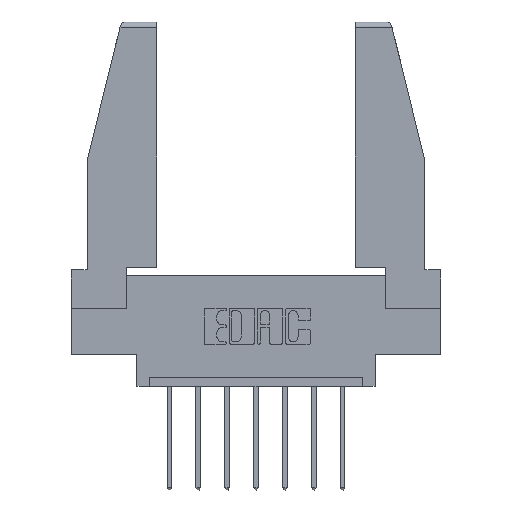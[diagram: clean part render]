
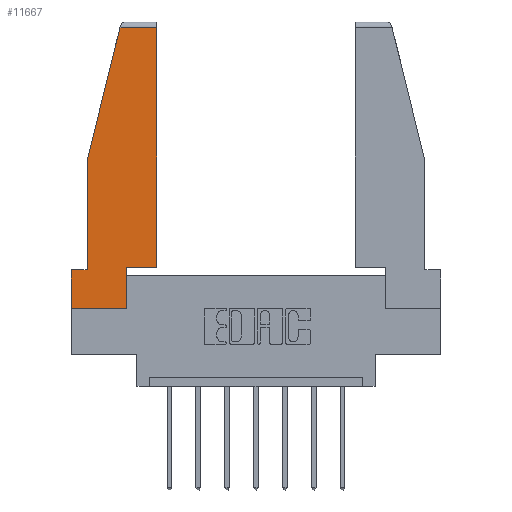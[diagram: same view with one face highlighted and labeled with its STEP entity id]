
A CAD part, top view. The second image highlights one B-rep face of the part: STEP entity #11667.
In plain terms, the highlighted planar face has unit normal (0, 0, 1).
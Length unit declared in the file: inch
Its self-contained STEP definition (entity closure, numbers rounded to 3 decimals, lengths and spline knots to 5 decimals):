
#62 = EDGE_CURVE ( 'NONE', #9672, #12344, #979, .T. ) ;
#103 = EDGE_CURVE ( 'NONE', #12301, #7534, #6642, .T. ) ;
#196 = LINE ( 'NONE', #8678, #3354 ) ;
#245 = DIRECTION ( 'NONE',  ( 1., 0., 0. ) ) ;
#257 = CARTESIAN_POINT ( 'NONE',  ( 0.297, 0., 0. ) ) ;
#567 = LINE ( 'NONE', #4056, #2531 ) ;
#785 = CARTESIAN_POINT ( 'NONE',  ( 0., 0.21, 0. ) ) ;
#924 = CARTESIAN_POINT ( 'NONE',  ( 0.271, 1.55, 0. ) ) ;
#925 = EDGE_CURVE ( 'NONE', #12068, #9672, #196, .T. ) ;
#979 = LINE ( 'NONE', #11365, #8722 ) ;
#1049 = DIRECTION ( 'NONE',  ( 0., 0., 1. ) ) ;
#1457 = VECTOR ( 'NONE', #11773, 39.37008 ) ;
#1503 = LINE ( 'NONE', #5486, #5255 ) ;
#1992 = CARTESIAN_POINT ( 'NONE',  ( 0.461, 0.223, 0. ) ) ;
#2228 = VERTEX_POINT ( 'NONE', #5398 ) ;
#2531 = VECTOR ( 'NONE', #245, 39.37008 ) ;
#2776 = ORIENTED_EDGE ( 'NONE', *, *, #9525, .T. ) ;
#2846 = EDGE_CURVE ( 'NONE', #2228, #6440, #1503, .T. ) ;
#2896 = ORIENTED_EDGE ( 'NONE', *, *, #11100, .T. ) ;
#3192 = CARTESIAN_POINT ( 'NONE',  ( 0., 0.21, 0. ) ) ;
#3193 = CARTESIAN_POINT ( 'NONE',  ( 0.461, 1.52, 0. ) ) ;
#3354 = VECTOR ( 'NONE', #9631, 39.37008 ) ;
#3935 = CARTESIAN_POINT ( 'NONE',  ( 0.086, 0.8, 0. ) ) ;
#3971 = DIRECTION ( 'NONE',  ( 0., 1., 0. ) ) ;
#3988 = LINE ( 'NONE', #924, #8746 ) ;
#4056 = CARTESIAN_POINT ( 'NONE',  ( 0.297, 0.223, 0. ) ) ;
#4350 = CARTESIAN_POINT ( 'NONE',  ( 0.086, 0.21, 0. ) ) ;
#4419 = ORIENTED_EDGE ( 'NONE', *, *, #11668, .T. ) ;
#4995 = CARTESIAN_POINT ( 'NONE',  ( 0., 0., 0. ) ) ;
#5255 = VECTOR ( 'NONE', #7343, 39.37008 ) ;
#5398 = CARTESIAN_POINT ( 'NONE',  ( 0., 0., 0. ) ) ;
#5486 = CARTESIAN_POINT ( 'NONE',  ( 0., 0., 0. ) ) ;
#5608 = ORIENTED_EDGE ( 'NONE', *, *, #8175, .T. ) ;
#5810 = VECTOR ( 'NONE', #11287, 39.37008 ) ;
#5862 = CARTESIAN_POINT ( 'NONE',  ( 0.2636, 1.52, 0. ) ) ;
#6181 = LINE ( 'NONE', #257, #10951 ) ;
#6210 = VERTEX_POINT ( 'NONE', #7979 ) ;
#6440 = VERTEX_POINT ( 'NONE', #7239 ) ;
#6583 = DIRECTION ( 'NONE',  ( -1., 0., 0. ) ) ;
#6642 = LINE ( 'NONE', #12356, #11411 ) ;
#7026 = ORIENTED_EDGE ( 'NONE', *, *, #103, .T. ) ;
#7239 = CARTESIAN_POINT ( 'NONE',  ( 0.297, 0., 0. ) ) ;
#7343 = DIRECTION ( 'NONE',  ( 1., 0., 0. ) ) ;
#7534 = VERTEX_POINT ( 'NONE', #4350 ) ;
#7979 = CARTESIAN_POINT ( 'NONE',  ( 0.297, 0.223, 0. ) ) ;
#8022 = ORIENTED_EDGE ( 'NONE', *, *, #2846, .T. ) ;
#8175 = EDGE_CURVE ( 'NONE', #12344, #12301, #3988, .T. ) ;
#8346 = LINE ( 'NONE', #785, #5810 ) ;
#8678 = CARTESIAN_POINT ( 'NONE',  ( 0.461, 0.223, 0. ) ) ;
#8722 = VECTOR ( 'NONE', #6583, 39.37008 ) ;
#8745 = DIRECTION ( 'NONE',  ( 1., 0., 0. ) ) ;
#8746 = VECTOR ( 'NONE', #11227, 39.37008 ) ;
#9195 = LINE ( 'NONE', #3192, #1457 ) ;
#9209 = FACE_OUTER_BOUND ( 'NONE', #11708, .T. ) ;
#9507 = DIRECTION ( 'NONE',  ( 0., -1., 0. ) ) ;
#9525 = EDGE_CURVE ( 'NONE', #6440, #6210, #6181, .T. ) ;
#9548 = CARTESIAN_POINT ( 'NONE',  ( 0., 0.21, 0. ) ) ;
#9602 = PLANE ( 'NONE',  #9778 ) ;
#9631 = DIRECTION ( 'NONE',  ( 0., 1., 0. ) ) ;
#9672 = VERTEX_POINT ( 'NONE', #3193 ) ;
#9769 = ORIENTED_EDGE ( 'NONE', *, *, #62, .T. ) ;
#9778 = AXIS2_PLACEMENT_3D ( 'NONE', #4995, #1049, #8745 ) ;
#9845 = ORIENTED_EDGE ( 'NONE', *, *, #925, .T. ) ;
#10951 = VECTOR ( 'NONE', #3971, 39.37008 ) ;
#11100 = EDGE_CURVE ( 'NONE', #12303, #2228, #8346, .T. ) ;
#11227 = DIRECTION ( 'NONE',  ( -0.239, -0.971, 0. ) ) ;
#11287 = DIRECTION ( 'NONE',  ( 0., -1., 0. ) ) ;
#11365 = CARTESIAN_POINT ( 'NONE',  ( 0., 1.52, 0. ) ) ;
#11411 = VECTOR ( 'NONE', #9507, 39.37008 ) ;
#11428 = ORIENTED_EDGE ( 'NONE', *, *, #11789, .T. ) ;
#11667 = ADVANCED_FACE ( 'NONE', ( #9209 ), #9602, .T. ) ;
#11668 = EDGE_CURVE ( 'NONE', #6210, #12068, #567, .T. ) ;
#11708 = EDGE_LOOP ( 'NONE', ( #9845, #9769, #5608, #7026, #11428, #2896, #8022, #2776, #4419 ) ) ;
#11773 = DIRECTION ( 'NONE',  ( -1., 0., 0. ) ) ;
#11789 = EDGE_CURVE ( 'NONE', #7534, #12303, #9195, .T. ) ;
#12068 = VERTEX_POINT ( 'NONE', #1992 ) ;
#12301 = VERTEX_POINT ( 'NONE', #3935 ) ;
#12303 = VERTEX_POINT ( 'NONE', #9548 ) ;
#12344 = VERTEX_POINT ( 'NONE', #5862 ) ;
#12356 = CARTESIAN_POINT ( 'NONE',  ( 0.086, 0.8, 0. ) ) ;
